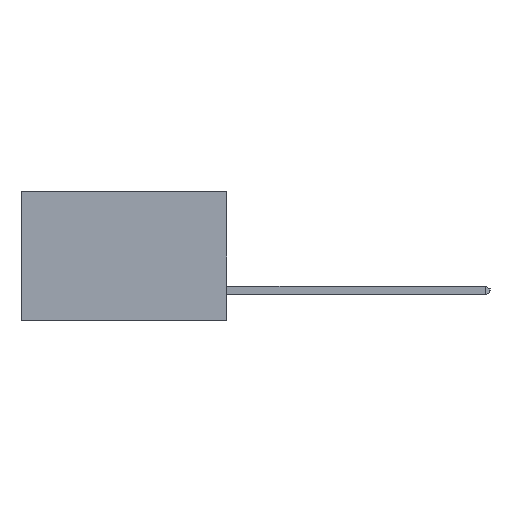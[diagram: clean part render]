
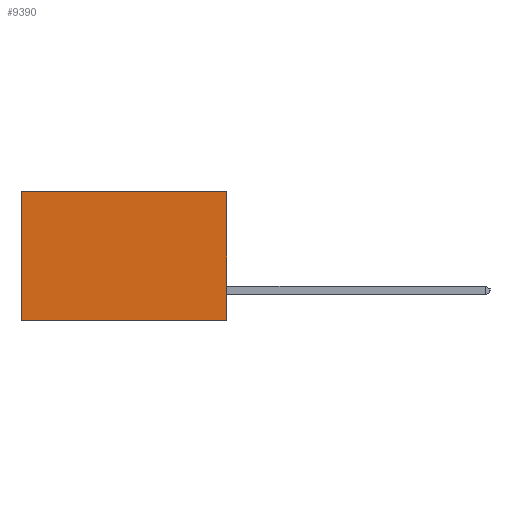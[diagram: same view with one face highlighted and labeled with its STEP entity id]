
A CAD part, left-side view. The second image highlights one B-rep face of the part: STEP entity #9390.
In plain terms, the highlighted planar face has unit normal (-1, 0, 0).
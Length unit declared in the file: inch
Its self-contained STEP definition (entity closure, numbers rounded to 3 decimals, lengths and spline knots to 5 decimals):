
#591 = VERTEX_POINT ( 'NONE', #10988 ) ;
#745 = VERTEX_POINT ( 'NONE', #6337 ) ;
#804 = VECTOR ( 'NONE', #1738, 39.37008 ) ;
#842 = CARTESIAN_POINT ( 'NONE',  ( 0.277, 0., 0. ) ) ;
#969 = DIRECTION ( 'NONE',  ( 0., 0., -1. ) ) ;
#1220 = CARTESIAN_POINT ( 'NONE',  ( 0.277, 0., -0.37 ) ) ;
#1292 = ORIENTED_EDGE ( 'NONE', *, *, #8228, .F. ) ;
#1425 = EDGE_LOOP ( 'NONE', ( #6586, #1292, #4365, #6388 ) ) ;
#1738 = DIRECTION ( 'NONE',  ( 0., 1., 0. ) ) ;
#2034 = LINE ( 'NONE', #6902, #4139 ) ;
#2366 = FACE_OUTER_BOUND ( 'NONE', #1425, .T. ) ;
#2897 = VERTEX_POINT ( 'NONE', #7572 ) ;
#2979 = DIRECTION ( 'NONE',  ( 0., 1., 0. ) ) ;
#3630 = LINE ( 'NONE', #8422, #7814 ) ;
#3636 = PLANE ( 'NONE',  #7234 ) ;
#4139 = VECTOR ( 'NONE', #7818, 39.37008 ) ;
#4365 = ORIENTED_EDGE ( 'NONE', *, *, #6196, .F. ) ;
#5247 = LINE ( 'NONE', #1220, #9723 ) ;
#5946 = VERTEX_POINT ( 'NONE', #8026 ) ;
#6196 = EDGE_CURVE ( 'NONE', #2897, #745, #3630, .T. ) ;
#6324 = DIRECTION ( 'NONE',  ( 1., 0., 0. ) ) ;
#6337 = CARTESIAN_POINT ( 'NONE',  ( 0.277, 0., -0.37 ) ) ;
#6388 = ORIENTED_EDGE ( 'NONE', *, *, #10170, .T. ) ;
#6586 = ORIENTED_EDGE ( 'NONE', *, *, #11220, .T. ) ;
#6902 = CARTESIAN_POINT ( 'NONE',  ( 0.277, 0.59, -0.37 ) ) ;
#7234 = AXIS2_PLACEMENT_3D ( 'NONE', #8970, #6324, #969 ) ;
#7572 = CARTESIAN_POINT ( 'NONE',  ( 0.277, 0., 0. ) ) ;
#7814 = VECTOR ( 'NONE', #9303, 39.37008 ) ;
#7818 = DIRECTION ( 'NONE',  ( 0., 0., -1. ) ) ;
#8026 = CARTESIAN_POINT ( 'NONE',  ( 0.277, 0.59, -0.37 ) ) ;
#8228 = EDGE_CURVE ( 'NONE', #745, #5946, #5247, .T. ) ;
#8422 = CARTESIAN_POINT ( 'NONE',  ( 0.277, 0., -0.37 ) ) ;
#8970 = CARTESIAN_POINT ( 'NONE',  ( 0.277, 0., -0.37 ) ) ;
#9303 = DIRECTION ( 'NONE',  ( 0., 0., -1. ) ) ;
#9390 = ADVANCED_FACE ( 'NONE', ( #2366 ), #3636, .F. ) ;
#9723 = VECTOR ( 'NONE', #2979, 39.37008 ) ;
#10170 = EDGE_CURVE ( 'NONE', #2897, #591, #10613, .T. ) ;
#10613 = LINE ( 'NONE', #842, #804 ) ;
#10988 = CARTESIAN_POINT ( 'NONE',  ( 0.277, 0.59, 0. ) ) ;
#11220 = EDGE_CURVE ( 'NONE', #591, #5946, #2034, .T. ) ;
